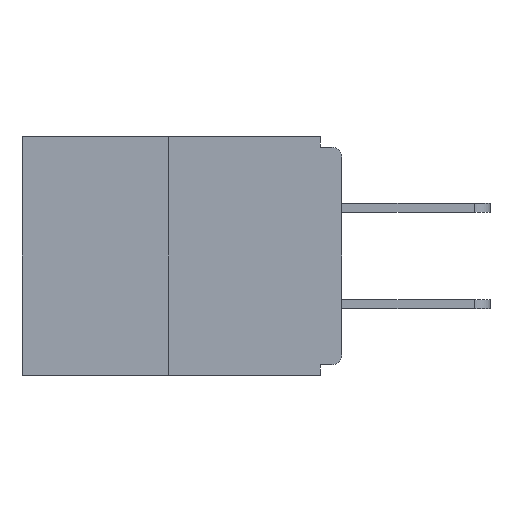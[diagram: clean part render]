
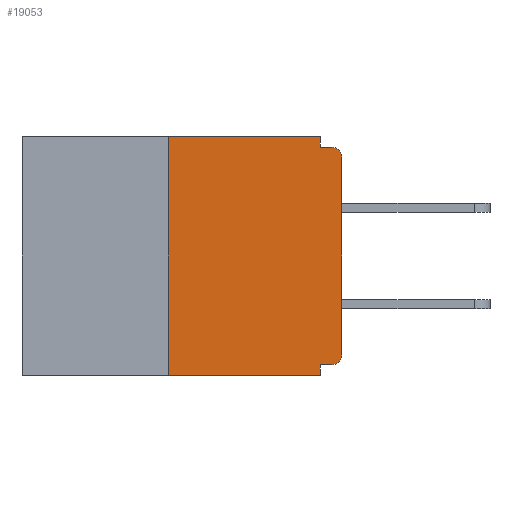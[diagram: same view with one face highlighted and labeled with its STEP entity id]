
A CAD part, left-side view. The second image highlights one B-rep face of the part: STEP entity #19053.
In plain terms, the highlighted planar face has unit normal (-1, 0, 0).
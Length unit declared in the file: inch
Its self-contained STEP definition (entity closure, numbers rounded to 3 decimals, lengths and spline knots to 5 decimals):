
#263 = CIRCLE ( 'NONE', #6637, 0.015 ) ;
#426 = EDGE_CURVE ( 'NONE', #16234, #2037, #5632, .T. ) ;
#534 = DIRECTION ( 'NONE',  ( 0., 0., -1. ) ) ;
#541 = DIRECTION ( 'NONE',  ( -1., 0., 0. ) ) ;
#702 = ORIENTED_EDGE ( 'NONE', *, *, #4345, .T. ) ;
#2037 = VERTEX_POINT ( 'NONE', #3436 ) ;
#2064 = AXIS2_PLACEMENT_3D ( 'NONE', #20899, #6961, #19129 ) ;
#2226 = CARTESIAN_POINT ( 'NONE',  ( 0., 0.015, -0.03 ) ) ;
#2341 = EDGE_CURVE ( 'NONE', #16266, #10365, #5025, .T. ) ;
#2495 = CARTESIAN_POINT ( 'NONE',  ( 0., 0.46, 0. ) ) ;
#2648 = VERTEX_POINT ( 'NONE', #16419 ) ;
#2890 = VERTEX_POINT ( 'NONE', #17526 ) ;
#3083 = DIRECTION ( 'NONE',  ( 0., 1., 0. ) ) ;
#3302 = LINE ( 'NONE', #6388, #18497 ) ;
#3436 = CARTESIAN_POINT ( 'NONE',  ( 0., 0.25, 0. ) ) ;
#4074 = ORIENTED_EDGE ( 'NONE', *, *, #13430, .T. ) ;
#4100 = CARTESIAN_POINT ( 'NONE',  ( 0., 0.031, 0. ) ) ;
#4345 = EDGE_CURVE ( 'NONE', #19362, #2890, #14206, .T. ) ;
#5025 = LINE ( 'NONE', #12587, #12927 ) ;
#5632 = LINE ( 'NONE', #19872, #18442 ) ;
#6007 = VECTOR ( 'NONE', #17403, 39.37008 ) ;
#6362 = CARTESIAN_POINT ( 'NONE',  ( 0., 0.015, -0.328 ) ) ;
#6388 = CARTESIAN_POINT ( 'NONE',  ( 0., 0., -0.328 ) ) ;
#6637 = AXIS2_PLACEMENT_3D ( 'NONE', #17809, #541, #12657 ) ;
#6961 = DIRECTION ( 'NONE',  ( 1., 0., 0. ) ) ;
#7254 = EDGE_CURVE ( 'NONE', #2648, #21863, #14205, .T. ) ;
#7662 = VERTEX_POINT ( 'NONE', #16441 ) ;
#8300 = CARTESIAN_POINT ( 'NONE',  ( 0., 0., -0.313 ) ) ;
#8408 = EDGE_CURVE ( 'NONE', #10365, #7662, #17163, .T. ) ;
#10103 = ORIENTED_EDGE ( 'NONE', *, *, #426, .F. ) ;
#10118 = VECTOR ( 'NONE', #19788, 39.37008 ) ;
#10365 = VERTEX_POINT ( 'NONE', #21353 ) ;
#10884 = ORIENTED_EDGE ( 'NONE', *, *, #22459, .T. ) ;
#11788 = DIRECTION ( 'NONE',  ( 0., -1., 0. ) ) ;
#11814 = DIRECTION ( 'NONE',  ( 0., -1., 0. ) ) ;
#11895 = LINE ( 'NONE', #2495, #20332 ) ;
#12228 = CARTESIAN_POINT ( 'NONE',  ( 0., 0., 0. ) ) ;
#12536 = VECTOR ( 'NONE', #11788, 39.37008 ) ;
#12587 = CARTESIAN_POINT ( 'NONE',  ( 0., 0.031, 0. ) ) ;
#12657 = DIRECTION ( 'NONE',  ( 0., 0., -1. ) ) ;
#12694 = ORIENTED_EDGE ( 'NONE', *, *, #8408, .F. ) ;
#12698 = LINE ( 'NONE', #13720, #20010 ) ;
#12793 = FACE_OUTER_BOUND ( 'NONE', #13115, .T. ) ;
#12859 = CARTESIAN_POINT ( 'NONE',  ( 0., 0.25, -0.343 ) ) ;
#12927 = VECTOR ( 'NONE', #14379, 39.37008 ) ;
#13115 = EDGE_LOOP ( 'NONE', ( #15099, #10103, #15636, #15035, #22028, #4074, #702, #10884, #12694, #21256 ) ) ;
#13430 = EDGE_CURVE ( 'NONE', #16336, #19362, #263, .T. ) ;
#13720 = CARTESIAN_POINT ( 'NONE',  ( 0., 0.46, -0.343 ) ) ;
#13970 = PLANE ( 'NONE',  #2064 ) ;
#14205 = LINE ( 'NONE', #19211, #6007 ) ;
#14206 = LINE ( 'NONE', #12228, #10118 ) ;
#14379 = DIRECTION ( 'NONE',  ( 0., 0., -1. ) ) ;
#14509 = DIRECTION ( 'NONE',  ( -1., 0., 0. ) ) ;
#14613 = DIRECTION ( 'NONE',  ( 0., 0., 1. ) ) ;
#15035 = ORIENTED_EDGE ( 'NONE', *, *, #7254, .F. ) ;
#15099 = ORIENTED_EDGE ( 'NONE', *, *, #15391, .F. ) ;
#15391 = EDGE_CURVE ( 'NONE', #2037, #16266, #11895, .T. ) ;
#15636 = ORIENTED_EDGE ( 'NONE', *, *, #21070, .T. ) ;
#16234 = VERTEX_POINT ( 'NONE', #12859 ) ;
#16266 = VERTEX_POINT ( 'NONE', #4100 ) ;
#16336 = VERTEX_POINT ( 'NONE', #6362 ) ;
#16419 = CARTESIAN_POINT ( 'NONE',  ( 0., 0.031, -0.328 ) ) ;
#16441 = CARTESIAN_POINT ( 'NONE',  ( 0., 0.015, -0.015 ) ) ;
#16642 = DIRECTION ( 'NONE',  ( 0., -1., 0. ) ) ;
#17163 = LINE ( 'NONE', #19910, #12536 ) ;
#17174 = CARTESIAN_POINT ( 'NONE',  ( 0., 0.031, -0.343 ) ) ;
#17403 = DIRECTION ( 'NONE',  ( 0., 0., -1. ) ) ;
#17526 = CARTESIAN_POINT ( 'NONE',  ( 0., 0., -0.03 ) ) ;
#17809 = CARTESIAN_POINT ( 'NONE',  ( 0., 0.015, -0.313 ) ) ;
#18442 = VECTOR ( 'NONE', #14613, 39.37008 ) ;
#18497 = VECTOR ( 'NONE', #3083, 39.37008 ) ;
#18623 = EDGE_CURVE ( 'NONE', #16336, #2648, #3302, .T. ) ;
#19053 = ADVANCED_FACE ( 'NONE', ( #12793 ), #13970, .F. ) ;
#19129 = DIRECTION ( 'NONE',  ( 0., 0., -1. ) ) ;
#19211 = CARTESIAN_POINT ( 'NONE',  ( 0., 0.031, -0.343 ) ) ;
#19362 = VERTEX_POINT ( 'NONE', #8300 ) ;
#19788 = DIRECTION ( 'NONE',  ( 0., 0., 1. ) ) ;
#19872 = CARTESIAN_POINT ( 'NONE',  ( 0., 0.25, 0. ) ) ;
#19910 = CARTESIAN_POINT ( 'NONE',  ( 0., 0., -0.015 ) ) ;
#20010 = VECTOR ( 'NONE', #11814, 39.37008 ) ;
#20332 = VECTOR ( 'NONE', #16642, 39.37008 ) ;
#20899 = CARTESIAN_POINT ( 'NONE',  ( 0., 0.46, 0. ) ) ;
#21070 = EDGE_CURVE ( 'NONE', #16234, #21863, #12698, .T. ) ;
#21256 = ORIENTED_EDGE ( 'NONE', *, *, #2341, .F. ) ;
#21349 = AXIS2_PLACEMENT_3D ( 'NONE', #2226, #14509, #534 ) ;
#21353 = CARTESIAN_POINT ( 'NONE',  ( 0., 0.031, -0.015 ) ) ;
#21598 = CIRCLE ( 'NONE', #21349, 0.015 ) ;
#21863 = VERTEX_POINT ( 'NONE', #17174 ) ;
#22028 = ORIENTED_EDGE ( 'NONE', *, *, #18623, .F. ) ;
#22459 = EDGE_CURVE ( 'NONE', #2890, #7662, #21598, .T. ) ;
